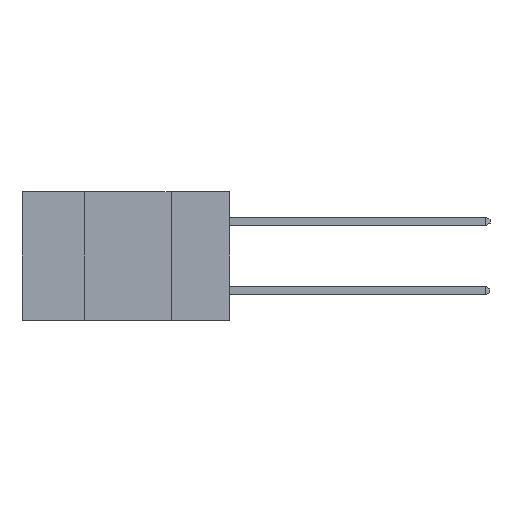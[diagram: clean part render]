
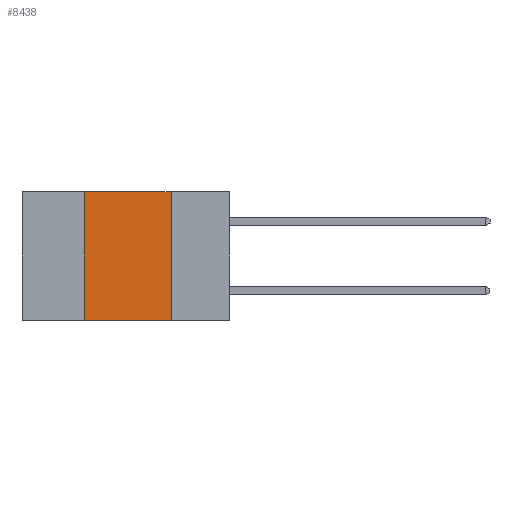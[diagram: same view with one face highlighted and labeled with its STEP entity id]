
A CAD part, left-side view. The second image highlights one B-rep face of the part: STEP entity #8438.
In plain terms, the highlighted planar face has unit normal (-1, 0, 0).
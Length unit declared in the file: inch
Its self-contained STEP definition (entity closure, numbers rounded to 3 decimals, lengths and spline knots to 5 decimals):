
#115 = VERTEX_POINT ( 'NONE', #3098 ) ;
#157 = LINE ( 'NONE', #5942, #7303 ) ;
#480 = CARTESIAN_POINT ( 'NONE',  ( 0., 0.42, -0.37 ) ) ;
#590 = EDGE_CURVE ( 'NONE', #9232, #3874, #11770, .T. ) ;
#962 = DIRECTION ( 'NONE',  ( 0., 0., 1. ) ) ;
#1030 = CARTESIAN_POINT ( 'NONE',  ( 0., 0.17, 0. ) ) ;
#1464 = CARTESIAN_POINT ( 'NONE',  ( 0., 0.6, 0. ) ) ;
#1493 = EDGE_CURVE ( 'NONE', #115, #9232, #9974, .T. ) ;
#1778 = DIRECTION ( 'NONE',  ( 0., 0., -1. ) ) ;
#2067 = CARTESIAN_POINT ( 'NONE',  ( 0., 0.17, -0.37 ) ) ;
#2079 = EDGE_CURVE ( 'NONE', #7729, #3874, #6873, .T. ) ;
#2195 = EDGE_CURVE ( 'NONE', #7729, #115, #157, .T. ) ;
#2461 = DIRECTION ( 'NONE',  ( 0., 0., -1. ) ) ;
#3098 = CARTESIAN_POINT ( 'NONE',  ( 0., 0.42, 0. ) ) ;
#3190 = FACE_OUTER_BOUND ( 'NONE', #7661, .T. ) ;
#3191 = DIRECTION ( 'NONE',  ( 0., -1., 0. ) ) ;
#3348 = PLANE ( 'NONE',  #8464 ) ;
#3874 = VERTEX_POINT ( 'NONE', #2067 ) ;
#4557 = ORIENTED_EDGE ( 'NONE', *, *, #590, .F. ) ;
#4656 = ORIENTED_EDGE ( 'NONE', *, *, #1493, .F. ) ;
#4909 = CARTESIAN_POINT ( 'NONE',  ( 0., 0.6, -0.37 ) ) ;
#4937 = ORIENTED_EDGE ( 'NONE', *, *, #2195, .F. ) ;
#5176 = ORIENTED_EDGE ( 'NONE', *, *, #2079, .T. ) ;
#5942 = CARTESIAN_POINT ( 'NONE',  ( 0., 0.42, 0. ) ) ;
#6592 = VECTOR ( 'NONE', #6939, 39.37008 ) ;
#6873 = LINE ( 'NONE', #4909, #6592 ) ;
#6939 = DIRECTION ( 'NONE',  ( 0., -1., 0. ) ) ;
#7077 = CARTESIAN_POINT ( 'NONE',  ( 0., 0.17, 0. ) ) ;
#7303 = VECTOR ( 'NONE', #962, 39.37008 ) ;
#7661 = EDGE_LOOP ( 'NONE', ( #4557, #4656, #4937, #5176 ) ) ;
#7729 = VERTEX_POINT ( 'NONE', #480 ) ;
#7917 = DIRECTION ( 'NONE',  ( 1., 0., 0. ) ) ;
#8438 = ADVANCED_FACE ( 'NONE', ( #3190 ), #3348, .F. ) ;
#8464 = AXIS2_PLACEMENT_3D ( 'NONE', #1464, #7917, #2461 ) ;
#9232 = VERTEX_POINT ( 'NONE', #7077 ) ;
#9379 = VECTOR ( 'NONE', #3191, 39.37008 ) ;
#9412 = VECTOR ( 'NONE', #1778, 39.37008 ) ;
#9974 = LINE ( 'NONE', #10571, #9379 ) ;
#10571 = CARTESIAN_POINT ( 'NONE',  ( 0., 0.6, 0. ) ) ;
#11770 = LINE ( 'NONE', #1030, #9412 ) ;
